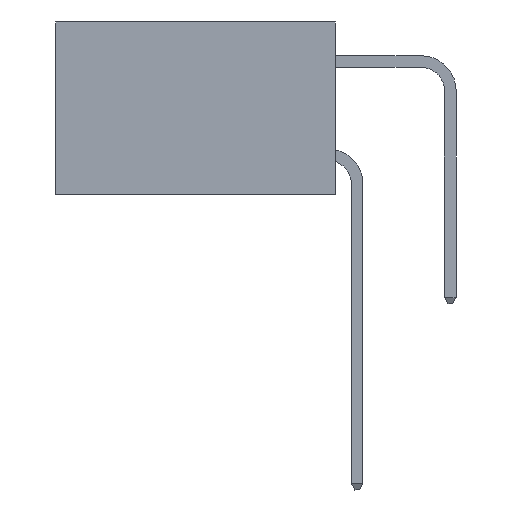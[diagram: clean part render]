
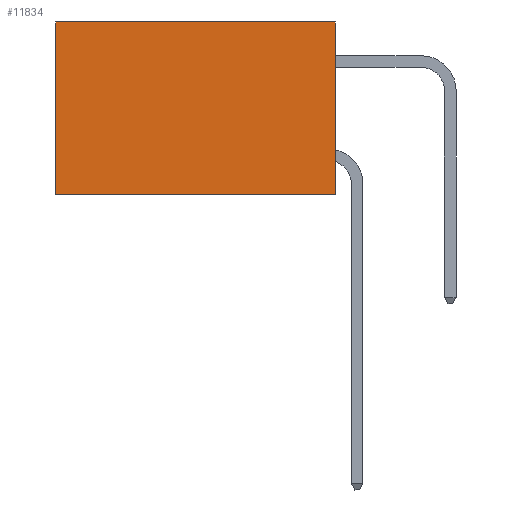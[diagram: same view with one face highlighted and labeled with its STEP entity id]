
A CAD part, left-side view. The second image highlights one B-rep face of the part: STEP entity #11834.
In plain terms, the highlighted planar face has unit normal (-1, 0, 0).
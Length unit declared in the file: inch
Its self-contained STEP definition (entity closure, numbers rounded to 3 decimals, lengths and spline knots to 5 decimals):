
#265 = DIRECTION ( 'NONE',  ( 0., 0., -1. ) ) ;
#668 = EDGE_LOOP ( 'NONE', ( #16176, #5785, #3473, #19925 ) ) ;
#1186 = FACE_OUTER_BOUND ( 'NONE', #668, .T. ) ;
#2901 = VECTOR ( 'NONE', #17963, 39.37008 ) ;
#3473 = ORIENTED_EDGE ( 'NONE', *, *, #11220, .F. ) ;
#5152 = VECTOR ( 'NONE', #5572, 39.37008 ) ;
#5329 = CARTESIAN_POINT ( 'NONE',  ( 0.2875, 0., 0. ) ) ;
#5418 = CARTESIAN_POINT ( 'NONE',  ( 0.2875, 0., -0.37 ) ) ;
#5488 = DIRECTION ( 'NONE',  ( 1., 0., 0. ) ) ;
#5572 = DIRECTION ( 'NONE',  ( 0., 0., -1. ) ) ;
#5785 = ORIENTED_EDGE ( 'NONE', *, *, #15102, .F. ) ;
#6091 = VERTEX_POINT ( 'NONE', #21881 ) ;
#6752 = LINE ( 'NONE', #19236, #15706 ) ;
#7294 = CARTESIAN_POINT ( 'NONE',  ( 0.2875, 0., 0. ) ) ;
#8548 = DIRECTION ( 'NONE',  ( 0., 1., 0. ) ) ;
#11139 = CARTESIAN_POINT ( 'NONE',  ( 0.2875, 0., 0. ) ) ;
#11220 = EDGE_CURVE ( 'NONE', #13729, #16428, #19229, .T. ) ;
#11834 = ADVANCED_FACE ( 'NONE', ( #1186 ), #23276, .F. ) ;
#13729 = VERTEX_POINT ( 'NONE', #5329 ) ;
#14534 = CARTESIAN_POINT ( 'NONE',  ( 0.2875, 0.6, 0. ) ) ;
#15102 = EDGE_CURVE ( 'NONE', #16428, #18646, #6752, .T. ) ;
#15643 = VECTOR ( 'NONE', #265, 39.37008 ) ;
#15706 = VECTOR ( 'NONE', #8548, 39.37008 ) ;
#16131 = CARTESIAN_POINT ( 'NONE',  ( 0.2875, 0.6, -0.37 ) ) ;
#16176 = ORIENTED_EDGE ( 'NONE', *, *, #21924, .T. ) ;
#16219 = CARTESIAN_POINT ( 'NONE',  ( 0.2875, 0., 0. ) ) ;
#16428 = VERTEX_POINT ( 'NONE', #5418 ) ;
#16694 = AXIS2_PLACEMENT_3D ( 'NONE', #16219, #5488, #17986 ) ;
#17242 = LINE ( 'NONE', #7294, #2901 ) ;
#17963 = DIRECTION ( 'NONE',  ( 0., 1., 0. ) ) ;
#17986 = DIRECTION ( 'NONE',  ( 0., 0., -1. ) ) ;
#18646 = VERTEX_POINT ( 'NONE', #16131 ) ;
#19229 = LINE ( 'NONE', #11139, #15643 ) ;
#19236 = CARTESIAN_POINT ( 'NONE',  ( 0.2875, 0., -0.37 ) ) ;
#19400 = LINE ( 'NONE', #14534, #5152 ) ;
#19925 = ORIENTED_EDGE ( 'NONE', *, *, #20695, .T. ) ;
#20695 = EDGE_CURVE ( 'NONE', #13729, #6091, #17242, .T. ) ;
#21881 = CARTESIAN_POINT ( 'NONE',  ( 0.2875, 0.6, 0. ) ) ;
#21924 = EDGE_CURVE ( 'NONE', #6091, #18646, #19400, .T. ) ;
#23276 = PLANE ( 'NONE',  #16694 ) ;
